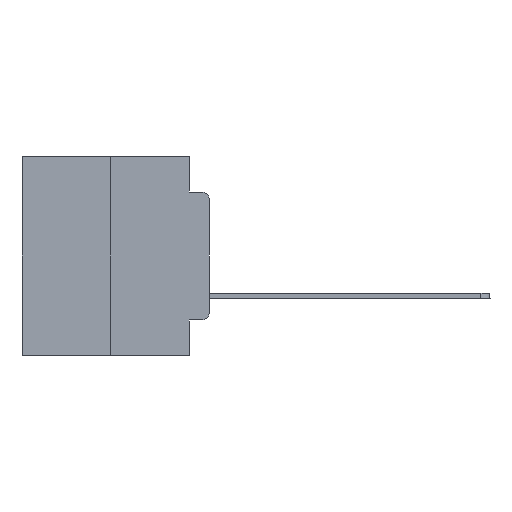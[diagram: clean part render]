
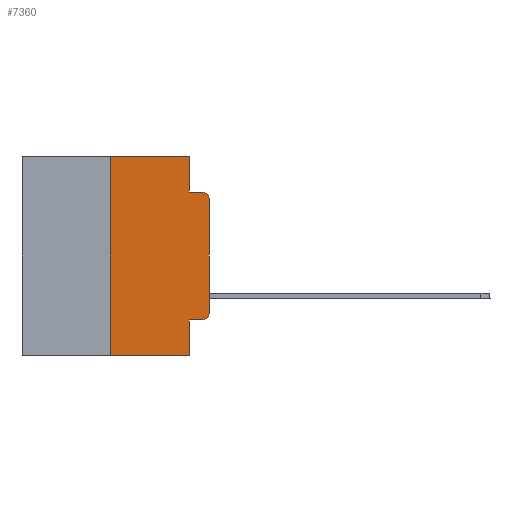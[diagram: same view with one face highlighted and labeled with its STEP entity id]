
A CAD part, left-side view. The second image highlights one B-rep face of the part: STEP entity #7360.
In plain terms, the highlighted planar face has unit normal (-1, 0, 0).
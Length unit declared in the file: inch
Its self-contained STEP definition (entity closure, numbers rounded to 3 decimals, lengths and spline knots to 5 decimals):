
#242 = VERTEX_POINT ( 'NONE', #10388 ) ;
#378 = LINE ( 'NONE', #17061, #4985 ) ;
#667 = CARTESIAN_POINT ( 'NONE',  ( 0., 0.25, 0. ) ) ;
#1370 = CARTESIAN_POINT ( 'NONE',  ( 0., 0.051, -0.0885 ) ) ;
#1411 = LINE ( 'NONE', #13524, #6342 ) ;
#1677 = DIRECTION ( 'NONE',  ( 0., -1., 0. ) ) ;
#1960 = CARTESIAN_POINT ( 'NONE',  ( 0., 0.02, -0.4115 ) ) ;
#2034 = DIRECTION ( 'NONE',  ( -1., 0., 0. ) ) ;
#2322 = DIRECTION ( 'NONE',  ( -1., 0., 0. ) ) ;
#2425 = ORIENTED_EDGE ( 'NONE', *, *, #8544, .T. ) ;
#2830 = VECTOR ( 'NONE', #15792, 39.37008 ) ;
#3301 = LINE ( 'NONE', #667, #19341 ) ;
#3383 = CARTESIAN_POINT ( 'NONE',  ( 0., 0.051, 0. ) ) ;
#3788 = EDGE_CURVE ( 'NONE', #14004, #5024, #21008, .T. ) ;
#3940 = ORIENTED_EDGE ( 'NONE', *, *, #16409, .F. ) ;
#4552 = DIRECTION ( 'NONE',  ( 0., 0., 1. ) ) ;
#4796 = DIRECTION ( 'NONE',  ( 0., -1., 0. ) ) ;
#4806 = AXIS2_PLACEMENT_3D ( 'NONE', #9824, #7892, #22433 ) ;
#4985 = VECTOR ( 'NONE', #4796, 39.37008 ) ;
#5024 = VERTEX_POINT ( 'NONE', #9560 ) ;
#5480 = LINE ( 'NONE', #3383, #27107 ) ;
#6342 = VECTOR ( 'NONE', #24064, 39.37008 ) ;
#6533 = DIRECTION ( 'NONE',  ( 0., 0., -1. ) ) ;
#6800 = CARTESIAN_POINT ( 'NONE',  ( 0., 0.02, -0.1085 ) ) ;
#7360 = ADVANCED_FACE ( 'NONE', ( #11662 ), #24652, .F. ) ;
#7892 = DIRECTION ( 'NONE',  ( 1., 0., 0. ) ) ;
#8097 = ORIENTED_EDGE ( 'NONE', *, *, #9978, .F. ) ;
#8544 = EDGE_CURVE ( 'NONE', #5024, #9024, #26348, .T. ) ;
#8841 = ORIENTED_EDGE ( 'NONE', *, *, #27054, .F. ) ;
#9024 = VERTEX_POINT ( 'NONE', #23731 ) ;
#9189 = VECTOR ( 'NONE', #25804, 39.37008 ) ;
#9344 = VECTOR ( 'NONE', #9396, 39.37008 ) ;
#9396 = DIRECTION ( 'NONE',  ( 0., 0., -1. ) ) ;
#9492 = CARTESIAN_POINT ( 'NONE',  ( 0., 0.25, 0. ) ) ;
#9560 = CARTESIAN_POINT ( 'NONE',  ( 0., 0., -0.1085 ) ) ;
#9782 = CARTESIAN_POINT ( 'NONE',  ( 0., 0.051, 0. ) ) ;
#9824 = CARTESIAN_POINT ( 'NONE',  ( 0., 0.473, 0. ) ) ;
#9899 = VERTEX_POINT ( 'NONE', #22020 ) ;
#9978 = EDGE_CURVE ( 'NONE', #26804, #10855, #5480, .T. ) ;
#10388 = CARTESIAN_POINT ( 'NONE',  ( 0., 0.051, -0.4115 ) ) ;
#10680 = ORIENTED_EDGE ( 'NONE', *, *, #24854, .T. ) ;
#10855 = VERTEX_POINT ( 'NONE', #1370 ) ;
#11662 = FACE_OUTER_BOUND ( 'NONE', #26679, .T. ) ;
#12280 = LINE ( 'NONE', #9782, #9344 ) ;
#12316 = LINE ( 'NONE', #22269, #2830 ) ;
#12803 = EDGE_CURVE ( 'NONE', #18558, #26804, #378, .T. ) ;
#13524 = CARTESIAN_POINT ( 'NONE',  ( 0., 0.473, -0.5 ) ) ;
#13735 = EDGE_CURVE ( 'NONE', #9899, #18558, #3301, .T. ) ;
#14004 = VERTEX_POINT ( 'NONE', #17159 ) ;
#15059 = VERTEX_POINT ( 'NONE', #21683 ) ;
#15306 = EDGE_CURVE ( 'NONE', #22966, #14004, #15322, .T. ) ;
#15322 = CIRCLE ( 'NONE', #25337, 0.02 ) ;
#15792 = DIRECTION ( 'NONE',  ( 0., -1., 0. ) ) ;
#16263 = ORIENTED_EDGE ( 'NONE', *, *, #3788, .T. ) ;
#16409 = EDGE_CURVE ( 'NONE', #242, #15059, #12280, .T. ) ;
#16415 = DIRECTION ( 'NONE',  ( 0., 0., -1. ) ) ;
#16554 = ORIENTED_EDGE ( 'NONE', *, *, #12803, .F. ) ;
#17061 = CARTESIAN_POINT ( 'NONE',  ( 0., 0.473, 0. ) ) ;
#17159 = CARTESIAN_POINT ( 'NONE',  ( 0., 0., -0.3915 ) ) ;
#17280 = CARTESIAN_POINT ( 'NONE',  ( 0., 0., 0. ) ) ;
#18145 = EDGE_CURVE ( 'NONE', #9899, #15059, #1411, .T. ) ;
#18558 = VERTEX_POINT ( 'NONE', #9492 ) ;
#19061 = ORIENTED_EDGE ( 'NONE', *, *, #13735, .F. ) ;
#19341 = VECTOR ( 'NONE', #4552, 39.37008 ) ;
#21008 = LINE ( 'NONE', #17280, #9189 ) ;
#21683 = CARTESIAN_POINT ( 'NONE',  ( 0., 0.051, -0.5 ) ) ;
#22020 = CARTESIAN_POINT ( 'NONE',  ( 0., 0.25, -0.5 ) ) ;
#22269 = CARTESIAN_POINT ( 'NONE',  ( 0., 0.051, -0.4115 ) ) ;
#22433 = DIRECTION ( 'NONE',  ( 0., 0., -1. ) ) ;
#22966 = VERTEX_POINT ( 'NONE', #1960 ) ;
#23633 = LINE ( 'NONE', #26808, #24326 ) ;
#23731 = CARTESIAN_POINT ( 'NONE',  ( 0., 0.02, -0.0885 ) ) ;
#24064 = DIRECTION ( 'NONE',  ( 0., -1., 0. ) ) ;
#24326 = VECTOR ( 'NONE', #1677, 39.37008 ) ;
#24652 = PLANE ( 'NONE',  #4806 ) ;
#24797 = ORIENTED_EDGE ( 'NONE', *, *, #18145, .T. ) ;
#24854 = EDGE_CURVE ( 'NONE', #242, #22966, #12316, .T. ) ;
#24879 = CARTESIAN_POINT ( 'NONE',  ( 0., 0.051, 0. ) ) ;
#25230 = ORIENTED_EDGE ( 'NONE', *, *, #15306, .T. ) ;
#25337 = AXIS2_PLACEMENT_3D ( 'NONE', #27129, #2034, #16415 ) ;
#25702 = AXIS2_PLACEMENT_3D ( 'NONE', #6800, #2322, #6533 ) ;
#25804 = DIRECTION ( 'NONE',  ( 0., 0., 1. ) ) ;
#26348 = CIRCLE ( 'NONE', #25702, 0.02 ) ;
#26548 = DIRECTION ( 'NONE',  ( 0., 0., -1. ) ) ;
#26679 = EDGE_LOOP ( 'NONE', ( #16263, #2425, #8841, #8097, #16554, #19061, #24797, #3940, #10680, #25230 ) ) ;
#26804 = VERTEX_POINT ( 'NONE', #24879 ) ;
#26808 = CARTESIAN_POINT ( 'NONE',  ( 0., 0.051, -0.0885 ) ) ;
#27054 = EDGE_CURVE ( 'NONE', #10855, #9024, #23633, .T. ) ;
#27107 = VECTOR ( 'NONE', #26548, 39.37008 ) ;
#27129 = CARTESIAN_POINT ( 'NONE',  ( 0., 0.02, -0.3915 ) ) ;
